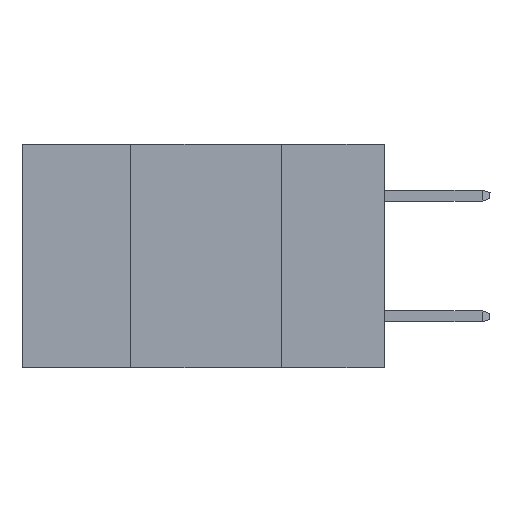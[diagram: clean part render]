
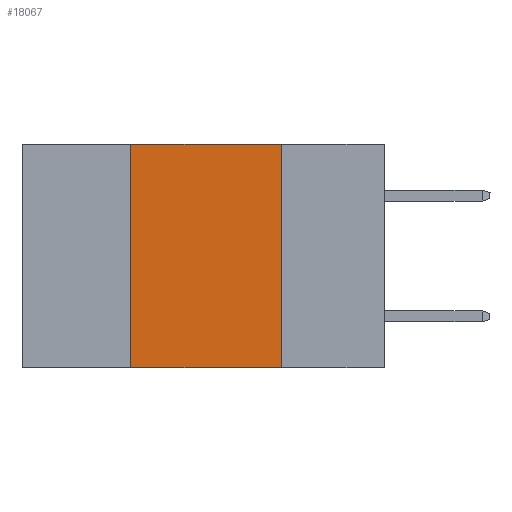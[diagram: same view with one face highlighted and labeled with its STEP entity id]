
A CAD part, left-side view. The second image highlights one B-rep face of the part: STEP entity #18067.
In plain terms, the highlighted planar face has unit normal (-1, 0, 0).
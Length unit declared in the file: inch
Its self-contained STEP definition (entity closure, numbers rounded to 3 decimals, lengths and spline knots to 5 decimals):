
#3569 = VECTOR ( 'NONE', #18573, 39.37008 ) ;
#4805 = ORIENTED_EDGE ( 'NONE', *, *, #16537, .F. ) ;
#4915 = CARTESIAN_POINT ( 'NONE',  ( 0., 0.6, 0. ) ) ;
#5388 = CARTESIAN_POINT ( 'NONE',  ( 0., 0.42, 0. ) ) ;
#6433 = CARTESIAN_POINT ( 'NONE',  ( 0., 0.42, -0.37 ) ) ;
#7024 = CARTESIAN_POINT ( 'NONE',  ( 0., 0.17, -0.37 ) ) ;
#8644 = DIRECTION ( 'NONE',  ( 0., 0., -1. ) ) ;
#10419 = PLANE ( 'NONE',  #19874 ) ;
#10597 = LINE ( 'NONE', #22411, #16044 ) ;
#10803 = DIRECTION ( 'NONE',  ( 0., -1., 0. ) ) ;
#12867 = ORIENTED_EDGE ( 'NONE', *, *, #14123, .F. ) ;
#13113 = CARTESIAN_POINT ( 'NONE',  ( 0., 0.17, -0.37 ) ) ;
#13139 = CARTESIAN_POINT ( 'NONE',  ( 0., 0.42, -0.37 ) ) ;
#13419 = DIRECTION ( 'NONE',  ( 0., -1., 0. ) ) ;
#14123 = EDGE_CURVE ( 'NONE', #21742, #22069, #14606, .T. ) ;
#14606 = LINE ( 'NONE', #13113, #3569 ) ;
#15098 = ORIENTED_EDGE ( 'NONE', *, *, #15338, .F. ) ;
#15338 = EDGE_CURVE ( 'NONE', #18266, #21742, #20915, .T. ) ;
#15561 = VECTOR ( 'NONE', #10803, 39.37008 ) ;
#16044 = VECTOR ( 'NONE', #13419, 39.37008 ) ;
#16537 = EDGE_CURVE ( 'NONE', #16969, #18266, #18094, .T. ) ;
#16969 = VERTEX_POINT ( 'NONE', #13139 ) ;
#17753 = EDGE_CURVE ( 'NONE', #16969, #22069, #10597, .T. ) ;
#18046 = ORIENTED_EDGE ( 'NONE', *, *, #17753, .T. ) ;
#18067 = ADVANCED_FACE ( 'NONE', ( #18301 ), #10419, .F. ) ;
#18094 = LINE ( 'NONE', #6433, #19226 ) ;
#18266 = VERTEX_POINT ( 'NONE', #5388 ) ;
#18301 = FACE_OUTER_BOUND ( 'NONE', #22454, .T. ) ;
#18573 = DIRECTION ( 'NONE',  ( 0., 0., -1. ) ) ;
#19226 = VECTOR ( 'NONE', #19269, 39.37008 ) ;
#19269 = DIRECTION ( 'NONE',  ( 0., 0., 1. ) ) ;
#19595 = DIRECTION ( 'NONE',  ( 1., 0., 0. ) ) ;
#19874 = AXIS2_PLACEMENT_3D ( 'NONE', #4915, #19595, #8644 ) ;
#19895 = CARTESIAN_POINT ( 'NONE',  ( 0., 0.6, 0. ) ) ;
#20695 = CARTESIAN_POINT ( 'NONE',  ( 0., 0.17, 0. ) ) ;
#20915 = LINE ( 'NONE', #19895, #15561 ) ;
#21742 = VERTEX_POINT ( 'NONE', #20695 ) ;
#22069 = VERTEX_POINT ( 'NONE', #7024 ) ;
#22411 = CARTESIAN_POINT ( 'NONE',  ( 0., 0.6, -0.37 ) ) ;
#22454 = EDGE_LOOP ( 'NONE', ( #12867, #15098, #4805, #18046 ) ) ;
